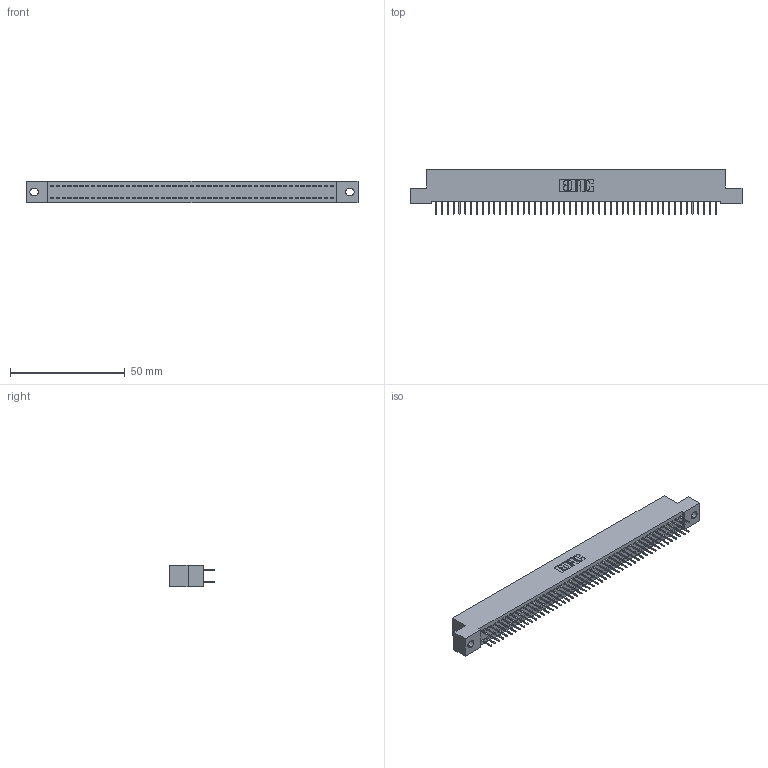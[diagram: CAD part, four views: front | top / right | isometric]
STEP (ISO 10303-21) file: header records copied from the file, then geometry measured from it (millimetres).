
FILE_DESCRIPTION (( 'STEP AP203' ), '1' );
FILE_NAME ('342-098-524-202.STEP', '2019-10-04T16:38:27', ( '' ), ( '' ), 'SwSTEP 2.0', 'SolidWorks 2016', '' );
FILE_SCHEMA (( 'CONFIG_CONTROL_DESIGN' ));
Length unit declared in the file: inch
Products named in the file (3): 342 Part_.128 Slot; 345-292-001_345-293-124; 342-098-524-202
Assembly tree (99 placements, depth 2):
  342-098-524-202
    342 Part_.128 Slot
    345-292-001_345-293-124  x98
Bounding box: 144.78 x 19.69 x 9.4 mm (x, y, z)
Volume: 12841.1 mm3; surface area: 20448.4 mm2
Topology: 99 solids, 99 shells, 5602 faces, 15893 edges, 10202 vertices
Faces by surface type: plane 4186, cylinder 1416
Entity records: 30695 total; most frequent: CARTESIAN_POINT 5078, ORIENTED_EDGE 5014, DIRECTION 4327, EDGE_CURVE 2507, VECTOR 2383, LINE 2383, VERTEX_POINT 1666, AXIS2_PLACEMENT_3D 972
